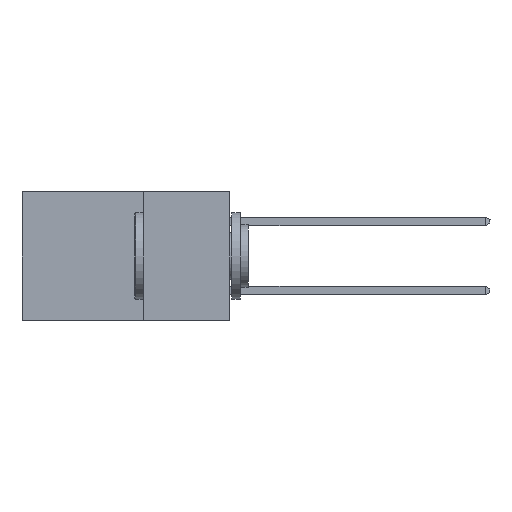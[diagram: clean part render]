
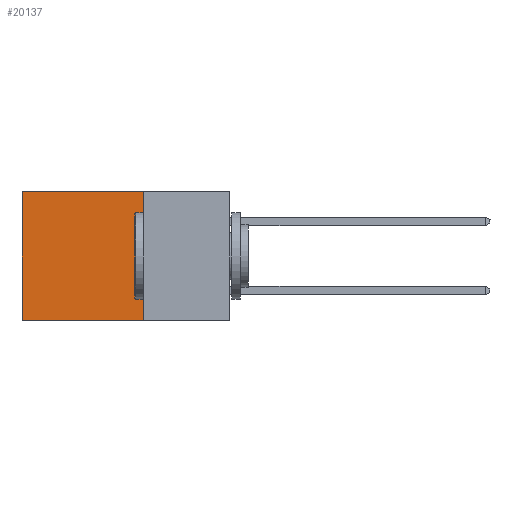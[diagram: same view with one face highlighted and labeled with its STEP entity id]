
A CAD part, left-side view. The second image highlights one B-rep face of the part: STEP entity #20137.
In plain terms, the highlighted planar face has unit normal (-1, 0, 0).
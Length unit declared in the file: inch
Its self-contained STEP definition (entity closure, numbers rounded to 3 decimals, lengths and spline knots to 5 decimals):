
#267 = LINE ( 'NONE', #7603, #21334 ) ;
#962 = VERTEX_POINT ( 'NONE', #17498 ) ;
#1067 = EDGE_CURVE ( 'NONE', #18865, #9330, #4384, .T. ) ;
#2233 = CARTESIAN_POINT ( 'NONE',  ( 0.2615, 0.25, -0.37 ) ) ;
#2572 = DIRECTION ( 'NONE',  ( 0., 0., -1. ) ) ;
#2911 = VECTOR ( 'NONE', #2572, 39.37008 ) ;
#3172 = ORIENTED_EDGE ( 'NONE', *, *, #7425, .F. ) ;
#4384 = LINE ( 'NONE', #18071, #11428 ) ;
#4813 = CARTESIAN_POINT ( 'NONE',  ( 0.2615, 0.6, 0. ) ) ;
#5299 = CARTESIAN_POINT ( 'NONE',  ( 0.2615, 0.25, 0. ) ) ;
#6306 = DIRECTION ( 'NONE',  ( 0., 0., -1. ) ) ;
#6635 = ORIENTED_EDGE ( 'NONE', *, *, #18119, .T. ) ;
#7425 = EDGE_CURVE ( 'NONE', #16823, #9330, #267, .T. ) ;
#7603 = CARTESIAN_POINT ( 'NONE',  ( 0.2615, 0.25, -0.37 ) ) ;
#8421 = EDGE_CURVE ( 'NONE', #962, #16823, #16145, .T. ) ;
#9330 = VERTEX_POINT ( 'NONE', #17887 ) ;
#10002 = AXIS2_PLACEMENT_3D ( 'NONE', #19936, #18452, #21760 ) ;
#11428 = VECTOR ( 'NONE', #6306, 39.37008 ) ;
#12405 = ORIENTED_EDGE ( 'NONE', *, *, #8421, .F. ) ;
#12816 = EDGE_LOOP ( 'NONE', ( #18731, #3172, #12405, #6635 ) ) ;
#14494 = DIRECTION ( 'NONE',  ( 0., 1., 0. ) ) ;
#14712 = PLANE ( 'NONE',  #10002 ) ;
#15812 = LINE ( 'NONE', #5299, #16451 ) ;
#16145 = LINE ( 'NONE', #2233, #2911 ) ;
#16451 = VECTOR ( 'NONE', #19107, 39.37008 ) ;
#16759 = FACE_OUTER_BOUND ( 'NONE', #12816, .T. ) ;
#16823 = VERTEX_POINT ( 'NONE', #20931 ) ;
#17498 = CARTESIAN_POINT ( 'NONE',  ( 0.2615, 0.25, 0. ) ) ;
#17887 = CARTESIAN_POINT ( 'NONE',  ( 0.2615, 0.6, -0.37 ) ) ;
#18071 = CARTESIAN_POINT ( 'NONE',  ( 0.2615, 0.6, -0.37 ) ) ;
#18119 = EDGE_CURVE ( 'NONE', #962, #18865, #15812, .T. ) ;
#18452 = DIRECTION ( 'NONE',  ( 1., 0., 0. ) ) ;
#18731 = ORIENTED_EDGE ( 'NONE', *, *, #1067, .T. ) ;
#18865 = VERTEX_POINT ( 'NONE', #4813 ) ;
#19107 = DIRECTION ( 'NONE',  ( 0., 1., 0. ) ) ;
#19936 = CARTESIAN_POINT ( 'NONE',  ( 0.2615, 0.25, -0.37 ) ) ;
#20137 = ADVANCED_FACE ( 'NONE', ( #16759 ), #14712, .F. ) ;
#20931 = CARTESIAN_POINT ( 'NONE',  ( 0.2615, 0.25, -0.37 ) ) ;
#21334 = VECTOR ( 'NONE', #14494, 39.37008 ) ;
#21760 = DIRECTION ( 'NONE',  ( 0., 0., -1. ) ) ;
